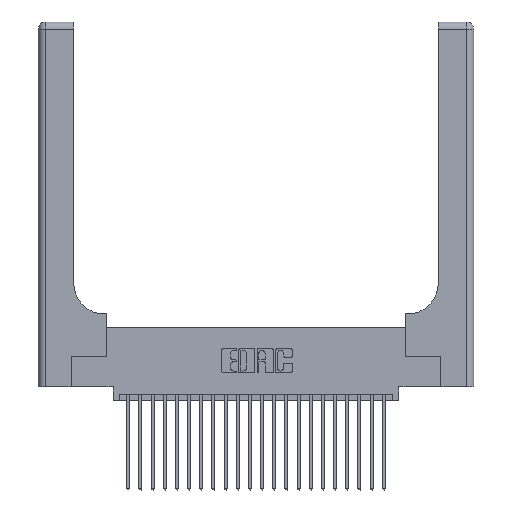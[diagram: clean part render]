
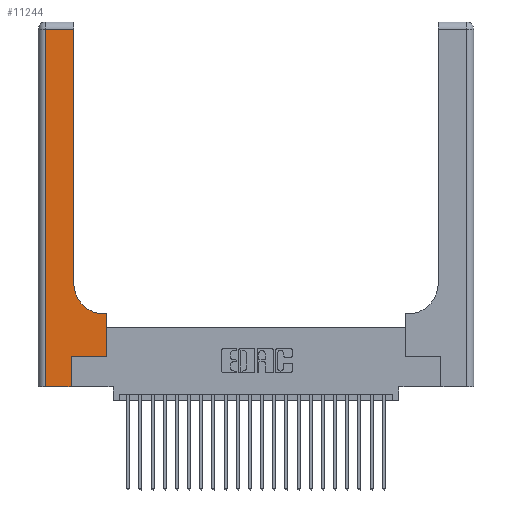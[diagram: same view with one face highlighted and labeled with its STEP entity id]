
A CAD part, top view. The second image highlights one B-rep face of the part: STEP entity #11244.
In plain terms, the highlighted planar face has unit normal (0, 0, 1).
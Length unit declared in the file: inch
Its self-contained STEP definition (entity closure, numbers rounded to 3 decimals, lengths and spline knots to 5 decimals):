
#46 = ORIENTED_EDGE ( 'NONE', *, *, #19145, .T. ) ;
#63 = CARTESIAN_POINT ( 'NONE',  ( 0.269, 0.25, 0.37 ) ) ;
#622 = LINE ( 'NONE', #19614, #24744 ) ;
#666 = ORIENTED_EDGE ( 'NONE', *, *, #18034, .T. ) ;
#907 = ORIENTED_EDGE ( 'NONE', *, *, #12277, .T. ) ;
#1304 = CARTESIAN_POINT ( 'NONE',  ( 0.269, 0.25, 0.37 ) ) ;
#2064 = LINE ( 'NONE', #2190, #17142 ) ;
#2190 = CARTESIAN_POINT ( 'NONE',  ( 0., 2.94, 0.37 ) ) ;
#2359 = DIRECTION ( 'NONE',  ( -1., 0., 0. ) ) ;
#2459 = VECTOR ( 'NONE', #15335, 39.37008 ) ;
#2886 = VERTEX_POINT ( 'NONE', #1304 ) ;
#3138 = EDGE_CURVE ( 'NONE', #3380, #13253, #2064, .T. ) ;
#3380 = VERTEX_POINT ( 'NONE', #20376 ) ;
#4226 = DIRECTION ( 'NONE',  ( -1., 0., 0. ) ) ;
#4947 = VECTOR ( 'NONE', #2359, 39.37008 ) ;
#5564 = VECTOR ( 'NONE', #7647, 39.37008 ) ;
#5665 = EDGE_CURVE ( 'NONE', #2886, #20246, #22625, .T. ) ;
#5736 = VERTEX_POINT ( 'NONE', #16358 ) ;
#6375 = CARTESIAN_POINT ( 'NONE',  ( 0.2915, 0.6, 0.37 ) ) ;
#6415 = ORIENTED_EDGE ( 'NONE', *, *, #7615, .T. ) ;
#6514 = ORIENTED_EDGE ( 'NONE', *, *, #18690, .T. ) ;
#6533 = CIRCLE ( 'NONE', #18701, 0.25 ) ;
#6620 = VECTOR ( 'NONE', #17432, 39.37008 ) ;
#6631 = EDGE_CURVE ( 'NONE', #20246, #16875, #18075, .T. ) ;
#7087 = LINE ( 'NONE', #11893, #16872 ) ;
#7615 = EDGE_CURVE ( 'NONE', #12730, #3380, #7087, .T. ) ;
#7647 = DIRECTION ( 'NONE',  ( 0., 1., 0. ) ) ;
#8034 = DIRECTION ( 'NONE',  ( -1., 0., 0. ) ) ;
#8505 = FACE_OUTER_BOUND ( 'NONE', #19599, .T. ) ;
#8543 = DIRECTION ( 'NONE',  ( 0., 0., -1. ) ) ;
#8602 = CARTESIAN_POINT ( 'NONE',  ( 0.269, 0., 0.37 ) ) ;
#9121 = ORIENTED_EDGE ( 'NONE', *, *, #3138, .T. ) ;
#10738 = LINE ( 'NONE', #17355, #5564 ) ;
#10764 = LINE ( 'NONE', #6375, #4947 ) ;
#11244 = ADVANCED_FACE ( 'NONE', ( #8505 ), #15836, .F. ) ;
#11825 = ORIENTED_EDGE ( 'NONE', *, *, #5665, .T. ) ;
#11893 = CARTESIAN_POINT ( 'NONE',  ( 0.2915, 3., 0.37 ) ) ;
#12277 = EDGE_CURVE ( 'NONE', #13755, #22838, #13078, .T. ) ;
#12391 = EDGE_CURVE ( 'NONE', #13253, #13755, #622, .T. ) ;
#12730 = VERTEX_POINT ( 'NONE', #15012 ) ;
#13078 = LINE ( 'NONE', #21208, #6620 ) ;
#13253 = VERTEX_POINT ( 'NONE', #24968 ) ;
#13350 = CARTESIAN_POINT ( 'NONE',  ( 0.5585, 0.25, 0.37 ) ) ;
#13755 = VERTEX_POINT ( 'NONE', #20794 ) ;
#13891 = DIRECTION ( 'NONE',  ( 0., 1., 0. ) ) ;
#14242 = AXIS2_PLACEMENT_3D ( 'NONE', #17724, #19669, #8034 ) ;
#14808 = CARTESIAN_POINT ( 'NONE',  ( 0.5585, 0.25, 0.37 ) ) ;
#15012 = CARTESIAN_POINT ( 'NONE',  ( 0.2915, 0.85, 0.37 ) ) ;
#15335 = DIRECTION ( 'NONE',  ( 0., 1., 0. ) ) ;
#15836 = PLANE ( 'NONE',  #14242 ) ;
#16358 = CARTESIAN_POINT ( 'NONE',  ( 0.5415, 0.6, 0.37 ) ) ;
#16872 = VECTOR ( 'NONE', #13891, 39.37008 ) ;
#16875 = VERTEX_POINT ( 'NONE', #18607 ) ;
#17142 = VECTOR ( 'NONE', #4226, 39.37008 ) ;
#17355 = CARTESIAN_POINT ( 'NONE',  ( 0.269, 0., 0.37 ) ) ;
#17432 = DIRECTION ( 'NONE',  ( 1., 0., 0. ) ) ;
#17552 = VECTOR ( 'NONE', #19778, 39.37008 ) ;
#17724 = CARTESIAN_POINT ( 'NONE',  ( 0., 3., 0.37 ) ) ;
#18034 = EDGE_CURVE ( 'NONE', #5736, #12730, #6533, .T. ) ;
#18075 = LINE ( 'NONE', #13350, #2459 ) ;
#18607 = CARTESIAN_POINT ( 'NONE',  ( 0.5585, 0.6, 0.37 ) ) ;
#18690 = EDGE_CURVE ( 'NONE', #16875, #5736, #10764, .T. ) ;
#18701 = AXIS2_PLACEMENT_3D ( 'NONE', #20155, #8543, #22081 ) ;
#19145 = EDGE_CURVE ( 'NONE', #22838, #2886, #10738, .T. ) ;
#19599 = EDGE_LOOP ( 'NONE', ( #6415, #9121, #21236, #907, #46, #11825, #20247, #6514, #666 ) ) ;
#19614 = CARTESIAN_POINT ( 'NONE',  ( 0.06, 3., 0.37 ) ) ;
#19669 = DIRECTION ( 'NONE',  ( 0., 0., -1. ) ) ;
#19778 = DIRECTION ( 'NONE',  ( 1., 0., 0. ) ) ;
#20155 = CARTESIAN_POINT ( 'NONE',  ( 0.5415, 0.85, 0.37 ) ) ;
#20246 = VERTEX_POINT ( 'NONE', #14808 ) ;
#20247 = ORIENTED_EDGE ( 'NONE', *, *, #6631, .T. ) ;
#20376 = CARTESIAN_POINT ( 'NONE',  ( 0.2915, 2.94, 0.37 ) ) ;
#20794 = CARTESIAN_POINT ( 'NONE',  ( 0.06, 0., 0.37 ) ) ;
#21208 = CARTESIAN_POINT ( 'NONE',  ( 0., 0., 0.37 ) ) ;
#21236 = ORIENTED_EDGE ( 'NONE', *, *, #12391, .T. ) ;
#21534 = DIRECTION ( 'NONE',  ( 0., -1., 0. ) ) ;
#22081 = DIRECTION ( 'NONE',  ( 1., 0., 0. ) ) ;
#22625 = LINE ( 'NONE', #63, #17552 ) ;
#22838 = VERTEX_POINT ( 'NONE', #8602 ) ;
#24744 = VECTOR ( 'NONE', #21534, 39.37008 ) ;
#24968 = CARTESIAN_POINT ( 'NONE',  ( 0.06, 2.94, 0.37 ) ) ;
